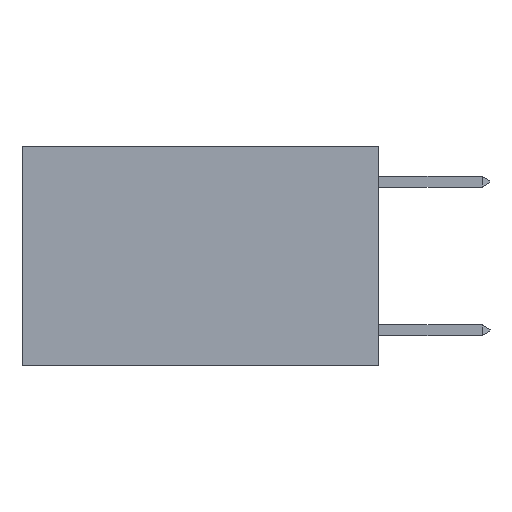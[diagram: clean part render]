
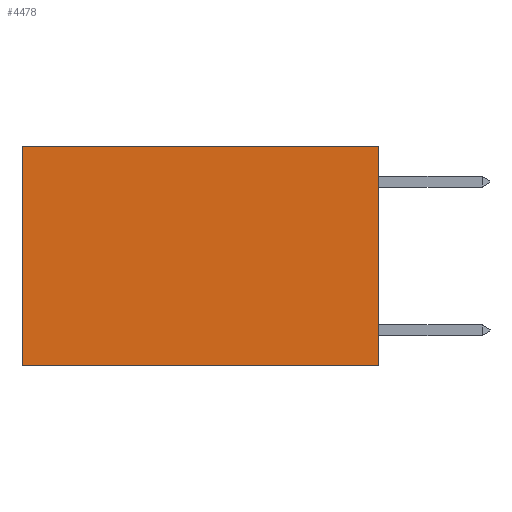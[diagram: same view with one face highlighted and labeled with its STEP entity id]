
A CAD part, left-side view. The second image highlights one B-rep face of the part: STEP entity #4478.
In plain terms, the highlighted planar face has unit normal (-1, 0, 0).
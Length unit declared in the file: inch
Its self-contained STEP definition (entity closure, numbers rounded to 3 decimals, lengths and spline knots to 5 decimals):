
#1312 = CARTESIAN_POINT ( 'NONE',  ( 0.2625, 0., 0. ) ) ;
#1576 = LINE ( 'NONE', #20235, #10218 ) ;
#3113 = DIRECTION ( 'NONE',  ( 0., 0., -1. ) ) ;
#3296 = VECTOR ( 'NONE', #11081, 39.37008 ) ;
#3537 = VERTEX_POINT ( 'NONE', #4014 ) ;
#3569 = VECTOR ( 'NONE', #21336, 39.37008 ) ;
#4014 = CARTESIAN_POINT ( 'NONE',  ( 0.2625, 0.6, -0.37 ) ) ;
#4478 = ADVANCED_FACE ( 'NONE', ( #15964 ), #18378, .F. ) ;
#5078 = VERTEX_POINT ( 'NONE', #11457 ) ;
#5147 = EDGE_LOOP ( 'NONE', ( #20272, #11214, #8965, #14927 ) ) ;
#5557 = EDGE_CURVE ( 'NONE', #5078, #19860, #12678, .T. ) ;
#7358 = LINE ( 'NONE', #21201, #3296 ) ;
#8408 = DIRECTION ( 'NONE',  ( 0., 0., -1. ) ) ;
#8644 = EDGE_CURVE ( 'NONE', #19860, #3537, #1576, .T. ) ;
#8858 = CARTESIAN_POINT ( 'NONE',  ( 0.2625, 0.6, 0. ) ) ;
#8965 = ORIENTED_EDGE ( 'NONE', *, *, #13863, .F. ) ;
#10218 = VECTOR ( 'NONE', #8408, 39.37008 ) ;
#10971 = AXIS2_PLACEMENT_3D ( 'NONE', #1312, #13367, #3113 ) ;
#10977 = EDGE_CURVE ( 'NONE', #13022, #3537, #17542, .T. ) ;
#11081 = DIRECTION ( 'NONE',  ( 0., 0., -1. ) ) ;
#11214 = ORIENTED_EDGE ( 'NONE', *, *, #10977, .F. ) ;
#11215 = CARTESIAN_POINT ( 'NONE',  ( 0.2625, 0., 0. ) ) ;
#11457 = CARTESIAN_POINT ( 'NONE',  ( 0.2625, 0., 0. ) ) ;
#12678 = LINE ( 'NONE', #11215, #3569 ) ;
#13022 = VERTEX_POINT ( 'NONE', #13631 ) ;
#13367 = DIRECTION ( 'NONE',  ( 1., 0., 0. ) ) ;
#13631 = CARTESIAN_POINT ( 'NONE',  ( 0.2625, 0., -0.37 ) ) ;
#13801 = DIRECTION ( 'NONE',  ( 0., 1., 0. ) ) ;
#13863 = EDGE_CURVE ( 'NONE', #5078, #13022, #7358, .T. ) ;
#14927 = ORIENTED_EDGE ( 'NONE', *, *, #5557, .T. ) ;
#15964 = FACE_OUTER_BOUND ( 'NONE', #5147, .T. ) ;
#17542 = LINE ( 'NONE', #18865, #21986 ) ;
#18378 = PLANE ( 'NONE',  #10971 ) ;
#18865 = CARTESIAN_POINT ( 'NONE',  ( 0.2625, 0., -0.37 ) ) ;
#19860 = VERTEX_POINT ( 'NONE', #8858 ) ;
#20235 = CARTESIAN_POINT ( 'NONE',  ( 0.2625, 0.6, 0. ) ) ;
#20272 = ORIENTED_EDGE ( 'NONE', *, *, #8644, .T. ) ;
#21201 = CARTESIAN_POINT ( 'NONE',  ( 0.2625, 0., 0. ) ) ;
#21336 = DIRECTION ( 'NONE',  ( 0., 1., 0. ) ) ;
#21986 = VECTOR ( 'NONE', #13801, 39.37008 ) ;
